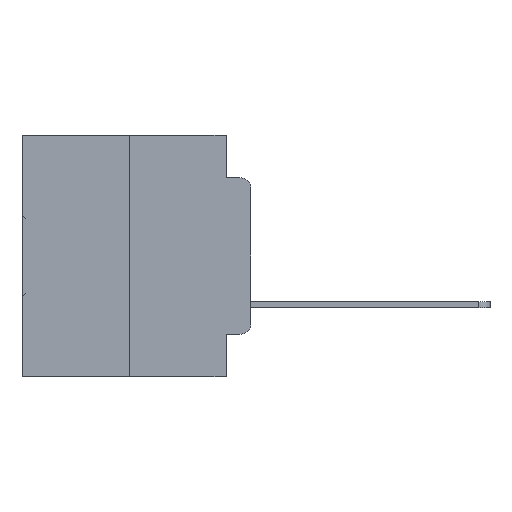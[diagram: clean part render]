
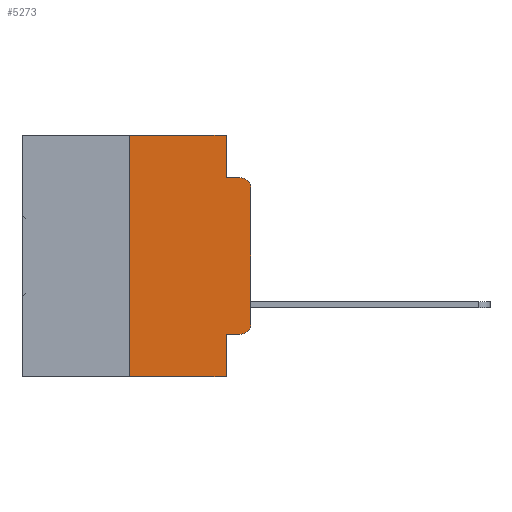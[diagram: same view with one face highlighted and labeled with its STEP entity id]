
A CAD part, left-side view. The second image highlights one B-rep face of the part: STEP entity #5273.
In plain terms, the highlighted planar face has unit normal (-1, 0, 0).
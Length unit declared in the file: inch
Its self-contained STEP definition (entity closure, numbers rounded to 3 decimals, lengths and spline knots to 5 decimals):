
#205 = DIRECTION ( 'NONE',  ( 0., 0., -1. ) ) ;
#819 = DIRECTION ( 'NONE',  ( 0., -1., 0. ) ) ;
#1445 = CARTESIAN_POINT ( 'NONE',  ( 0., 0.02, -0.0885 ) ) ;
#1670 = CARTESIAN_POINT ( 'NONE',  ( 0., 0., -0.1085 ) ) ;
#1803 = CARTESIAN_POINT ( 'NONE',  ( 0., 0., 0. ) ) ;
#2066 = CARTESIAN_POINT ( 'NONE',  ( 0., 0.25, 0. ) ) ;
#2698 = DIRECTION ( 'NONE',  ( 0., 0., -1. ) ) ;
#3086 = CARTESIAN_POINT ( 'NONE',  ( 0., 0.051, 0. ) ) ;
#3535 = EDGE_CURVE ( 'NONE', #18866, #10952, #17929, .T. ) ;
#3714 = DIRECTION ( 'NONE',  ( -1., 0., 0. ) ) ;
#3867 = AXIS2_PLACEMENT_3D ( 'NONE', #33203, #17493, #205 ) ;
#4177 = CARTESIAN_POINT ( 'NONE',  ( 0., 0.051, -0.5 ) ) ;
#4319 = LINE ( 'NONE', #12855, #11101 ) ;
#4417 = VERTEX_POINT ( 'NONE', #21310 ) ;
#4555 = LINE ( 'NONE', #2066, #32631 ) ;
#5273 = ADVANCED_FACE ( 'NONE', ( #21979 ), #11276, .F. ) ;
#5381 = DIRECTION ( 'NONE',  ( 0., -1., 0. ) ) ;
#5725 = CARTESIAN_POINT ( 'NONE',  ( 0., 0.051, -0.0885 ) ) ;
#8703 = VERTEX_POINT ( 'NONE', #4177 ) ;
#8907 = EDGE_CURVE ( 'NONE', #4417, #24291, #4555, .T. ) ;
#8968 = ORIENTED_EDGE ( 'NONE', *, *, #9649, .F. ) ;
#9413 = ORIENTED_EDGE ( 'NONE', *, *, #21866, .F. ) ;
#9649 = EDGE_CURVE ( 'NONE', #25531, #8703, #19076, .T. ) ;
#9734 = CARTESIAN_POINT ( 'NONE',  ( 0., 0.051, 0. ) ) ;
#10099 = CARTESIAN_POINT ( 'NONE',  ( 0., 0.051, -0.4115 ) ) ;
#10499 = VECTOR ( 'NONE', #34542, 39.37008 ) ;
#10952 = VERTEX_POINT ( 'NONE', #1670 ) ;
#11101 = VECTOR ( 'NONE', #21066, 39.37008 ) ;
#11276 = PLANE ( 'NONE',  #21668 ) ;
#12855 = CARTESIAN_POINT ( 'NONE',  ( 0., 0.051, 0. ) ) ;
#13316 = VECTOR ( 'NONE', #819, 39.37008 ) ;
#14536 = VECTOR ( 'NONE', #33812, 39.37008 ) ;
#14628 = EDGE_CURVE ( 'NONE', #24291, #28369, #21921, .T. ) ;
#15173 = ORIENTED_EDGE ( 'NONE', *, *, #3535, .T. ) ;
#16480 = ORIENTED_EDGE ( 'NONE', *, *, #25022, .T. ) ;
#16531 = DIRECTION ( 'NONE',  ( 0., 0., 1. ) ) ;
#17033 = CARTESIAN_POINT ( 'NONE',  ( 0., 0.473, 0. ) ) ;
#17374 = EDGE_LOOP ( 'NONE', ( #15173, #22314, #9413, #17734, #19419, #21090, #28933, #8968, #16480, #32555 ) ) ;
#17493 = DIRECTION ( 'NONE',  ( -1., 0., 0. ) ) ;
#17734 = ORIENTED_EDGE ( 'NONE', *, *, #18315, .F. ) ;
#17929 = LINE ( 'NONE', #1803, #10499 ) ;
#17999 = CARTESIAN_POINT ( 'NONE',  ( 0., 0., -0.3915 ) ) ;
#18315 = EDGE_CURVE ( 'NONE', #28369, #21368, #4319, .T. ) ;
#18856 = CIRCLE ( 'NONE', #3867, 0.02 ) ;
#18866 = VERTEX_POINT ( 'NONE', #17999 ) ;
#19076 = LINE ( 'NONE', #3086, #25333 ) ;
#19419 = ORIENTED_EDGE ( 'NONE', *, *, #14628, .F. ) ;
#19423 = EDGE_CURVE ( 'NONE', #10952, #19563, #18856, .T. ) ;
#19563 = VERTEX_POINT ( 'NONE', #1445 ) ;
#19723 = DIRECTION ( 'NONE',  ( 0., 0., -1. ) ) ;
#19767 = CIRCLE ( 'NONE', #22672, 0.02 ) ;
#20587 = CARTESIAN_POINT ( 'NONE',  ( 0., 0.02, -0.3915 ) ) ;
#21066 = DIRECTION ( 'NONE',  ( 0., 0., -1. ) ) ;
#21090 = ORIENTED_EDGE ( 'NONE', *, *, #8907, .F. ) ;
#21310 = CARTESIAN_POINT ( 'NONE',  ( 0., 0.25, -0.5 ) ) ;
#21368 = VERTEX_POINT ( 'NONE', #5725 ) ;
#21668 = AXIS2_PLACEMENT_3D ( 'NONE', #17033, #35333, #19723 ) ;
#21866 = EDGE_CURVE ( 'NONE', #21368, #19563, #24414, .T. ) ;
#21921 = LINE ( 'NONE', #35019, #27303 ) ;
#21979 = FACE_OUTER_BOUND ( 'NONE', #17374, .T. ) ;
#22203 = EDGE_CURVE ( 'NONE', #23022, #18866, #19767, .T. ) ;
#22314 = ORIENTED_EDGE ( 'NONE', *, *, #19423, .T. ) ;
#22672 = AXIS2_PLACEMENT_3D ( 'NONE', #20587, #3714, #23286 ) ;
#22693 = VECTOR ( 'NONE', #27020, 39.37008 ) ;
#23022 = VERTEX_POINT ( 'NONE', #32834 ) ;
#23286 = DIRECTION ( 'NONE',  ( 0., 0., -1. ) ) ;
#24291 = VERTEX_POINT ( 'NONE', #28152 ) ;
#24414 = LINE ( 'NONE', #34753, #22693 ) ;
#25022 = EDGE_CURVE ( 'NONE', #25531, #23022, #29094, .T. ) ;
#25333 = VECTOR ( 'NONE', #2698, 39.37008 ) ;
#25531 = VERTEX_POINT ( 'NONE', #10099 ) ;
#26088 = CARTESIAN_POINT ( 'NONE',  ( 0., 0.051, -0.4115 ) ) ;
#27020 = DIRECTION ( 'NONE',  ( 0., -1., 0. ) ) ;
#27303 = VECTOR ( 'NONE', #5381, 39.37008 ) ;
#27607 = LINE ( 'NONE', #33711, #13316 ) ;
#28152 = CARTESIAN_POINT ( 'NONE',  ( 0., 0.25, 0. ) ) ;
#28369 = VERTEX_POINT ( 'NONE', #9734 ) ;
#28933 = ORIENTED_EDGE ( 'NONE', *, *, #33581, .T. ) ;
#29094 = LINE ( 'NONE', #26088, #14536 ) ;
#32555 = ORIENTED_EDGE ( 'NONE', *, *, #22203, .T. ) ;
#32631 = VECTOR ( 'NONE', #16531, 39.37008 ) ;
#32834 = CARTESIAN_POINT ( 'NONE',  ( 0., 0.02, -0.4115 ) ) ;
#33203 = CARTESIAN_POINT ( 'NONE',  ( 0., 0.02, -0.1085 ) ) ;
#33581 = EDGE_CURVE ( 'NONE', #4417, #8703, #27607, .T. ) ;
#33711 = CARTESIAN_POINT ( 'NONE',  ( 0., 0.473, -0.5 ) ) ;
#33812 = DIRECTION ( 'NONE',  ( 0., -1., 0. ) ) ;
#34542 = DIRECTION ( 'NONE',  ( 0., 0., 1. ) ) ;
#34753 = CARTESIAN_POINT ( 'NONE',  ( 0., 0.051, -0.0885 ) ) ;
#35019 = CARTESIAN_POINT ( 'NONE',  ( 0., 0.473, 0. ) ) ;
#35333 = DIRECTION ( 'NONE',  ( 1., 0., 0. ) ) ;
